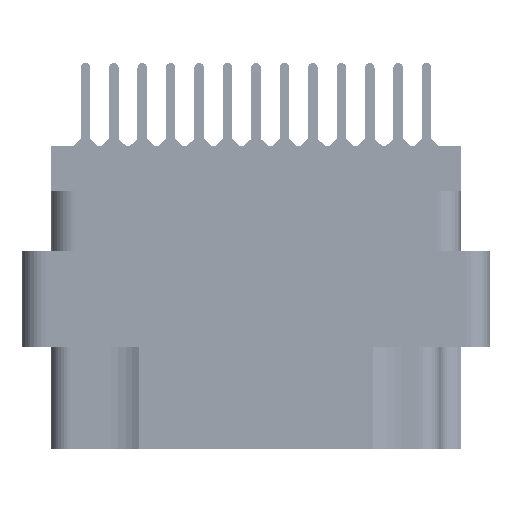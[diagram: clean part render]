
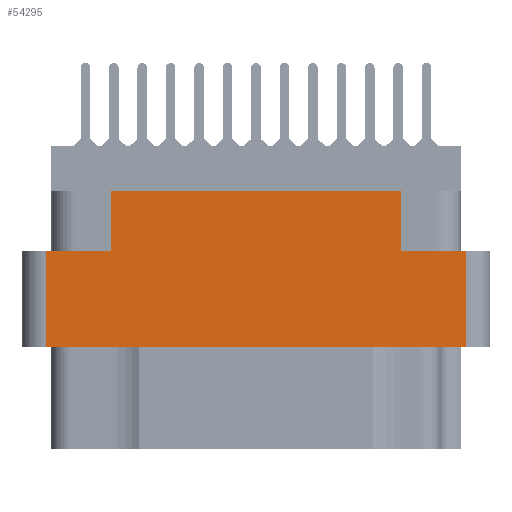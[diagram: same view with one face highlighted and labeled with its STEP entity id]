
A CAD part, left-side view. The second image highlights one B-rep face of the part: STEP entity #54295.
In plain terms, the highlighted planar face has unit normal (-1, 0, 0).
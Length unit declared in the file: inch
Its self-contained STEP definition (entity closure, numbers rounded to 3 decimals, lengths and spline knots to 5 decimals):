
#171 = DIRECTION ( 'NONE',  ( 0., 0., 1. ) ) ;
#1696 = LINE ( 'NONE', #37848, #60438 ) ;
#2802 = CARTESIAN_POINT ( 'NONE',  ( -1.359, -0.555, -0.798 ) ) ;
#3169 = VERTEX_POINT ( 'NONE', #52863 ) ;
#4063 = CARTESIAN_POINT ( 'NONE',  ( -1.359, 0.555, -0.798 ) ) ;
#6228 = LINE ( 'NONE', #41258, #57355 ) ;
#6602 = CARTESIAN_POINT ( 'NONE',  ( -1.359, -0.3825, -0.277 ) ) ;
#6632 = ORIENTED_EDGE ( 'NONE', *, *, #34053, .F. ) ;
#7445 = CARTESIAN_POINT ( 'NONE',  ( -1.359, -0.555, -0.277 ) ) ;
#7615 = ORIENTED_EDGE ( 'NONE', *, *, #39332, .F. ) ;
#7679 = VERTEX_POINT ( 'NONE', #59091 ) ;
#8671 = CARTESIAN_POINT ( 'NONE',  ( -1.359, 0.555, -0.529 ) ) ;
#9041 = DIRECTION ( 'NONE',  ( 0., 0., 1. ) ) ;
#10512 = EDGE_CURVE ( 'NONE', #35451, #7679, #48412, .T. ) ;
#11141 = LINE ( 'NONE', #4063, #49497 ) ;
#13252 = AXIS2_PLACEMENT_3D ( 'NONE', #14838, #52762, #20114 ) ;
#13747 = EDGE_CURVE ( 'NONE', #23393, #40418, #6228, .T. ) ;
#14532 = DIRECTION ( 'NONE',  ( 0., 0., -1. ) ) ;
#14607 = PLANE ( 'NONE',  #13252 ) ;
#14838 = CARTESIAN_POINT ( 'NONE',  ( -1.359, -0.617, -0.798 ) ) ;
#17220 = VERTEX_POINT ( 'NONE', #7445 ) ;
#19084 = LINE ( 'NONE', #23285, #31061 ) ;
#20112 = EDGE_CURVE ( 'NONE', #23393, #17220, #23311, .T. ) ;
#20114 = DIRECTION ( 'NONE',  ( 0., 0., 1. ) ) ;
#20311 = EDGE_CURVE ( 'NONE', #35451, #17220, #59917, .T. ) ;
#23285 = CARTESIAN_POINT ( 'NONE',  ( -1.359, 0., -0.277 ) ) ;
#23311 = LINE ( 'NONE', #2802, #70153 ) ;
#23393 = VERTEX_POINT ( 'NONE', #26243 ) ;
#26243 = CARTESIAN_POINT ( 'NONE',  ( -1.359, -0.555, -0.529 ) ) ;
#28966 = ORIENTED_EDGE ( 'NONE', *, *, #10512, .T. ) ;
#29539 = EDGE_LOOP ( 'NONE', ( #6632, #41146, #60265, #61091, #62860, #28966, #7615, #56392 ) ) ;
#30198 = VERTEX_POINT ( 'NONE', #33476 ) ;
#31061 = VECTOR ( 'NONE', #45719, 39.37008 ) ;
#33433 = VERTEX_POINT ( 'NONE', #57654 ) ;
#33476 = CARTESIAN_POINT ( 'NONE',  ( -1.359, 0.555, -0.277 ) ) ;
#34053 = EDGE_CURVE ( 'NONE', #30198, #33433, #19084, .T. ) ;
#35451 = VERTEX_POINT ( 'NONE', #6602 ) ;
#37834 = CARTESIAN_POINT ( 'NONE',  ( -1.359, 0., -0.277 ) ) ;
#37848 = CARTESIAN_POINT ( 'NONE',  ( -1.359, 0.617, -0.117 ) ) ;
#38007 = EDGE_CURVE ( 'NONE', #33433, #3169, #68318, .T. ) ;
#39332 = EDGE_CURVE ( 'NONE', #3169, #7679, #1696, .T. ) ;
#40418 = VERTEX_POINT ( 'NONE', #8671 ) ;
#41146 = ORIENTED_EDGE ( 'NONE', *, *, #47521, .T. ) ;
#41258 = CARTESIAN_POINT ( 'NONE',  ( -1.359, 0., -0.529 ) ) ;
#43101 = DIRECTION ( 'NONE',  ( 0., -1., 0. ) ) ;
#44653 = VECTOR ( 'NONE', #70182, 39.37008 ) ;
#45719 = DIRECTION ( 'NONE',  ( 0., -1., 0. ) ) ;
#46242 = VECTOR ( 'NONE', #171, 39.37008 ) ;
#47521 = EDGE_CURVE ( 'NONE', #30198, #40418, #11141, .T. ) ;
#48412 = LINE ( 'NONE', #62634, #67168 ) ;
#49497 = VECTOR ( 'NONE', #14532, 39.37008 ) ;
#51963 = DIRECTION ( 'NONE',  ( 0., 0., 1. ) ) ;
#52504 = FACE_OUTER_BOUND ( 'NONE', #29539, .T. ) ;
#52762 = DIRECTION ( 'NONE',  ( -1., 0., 0. ) ) ;
#52863 = CARTESIAN_POINT ( 'NONE',  ( -1.359, 0.3825, -0.117 ) ) ;
#54021 = CARTESIAN_POINT ( 'NONE',  ( -1.359, 0.3825, -0.277 ) ) ;
#54295 = ADVANCED_FACE ( 'NONE', ( #52504 ), #14607, .T. ) ;
#56392 = ORIENTED_EDGE ( 'NONE', *, *, #38007, .F. ) ;
#56946 = DIRECTION ( 'NONE',  ( 0., 1., 0. ) ) ;
#57355 = VECTOR ( 'NONE', #56946, 39.37008 ) ;
#57654 = CARTESIAN_POINT ( 'NONE',  ( -1.359, 0.3825, -0.277 ) ) ;
#59091 = CARTESIAN_POINT ( 'NONE',  ( -1.359, -0.3825, -0.117 ) ) ;
#59917 = LINE ( 'NONE', #37834, #44653 ) ;
#60265 = ORIENTED_EDGE ( 'NONE', *, *, #13747, .F. ) ;
#60438 = VECTOR ( 'NONE', #43101, 39.37008 ) ;
#61091 = ORIENTED_EDGE ( 'NONE', *, *, #20112, .T. ) ;
#62634 = CARTESIAN_POINT ( 'NONE',  ( -1.359, -0.3825, -0.277 ) ) ;
#62860 = ORIENTED_EDGE ( 'NONE', *, *, #20311, .F. ) ;
#67168 = VECTOR ( 'NONE', #51963, 39.37008 ) ;
#68318 = LINE ( 'NONE', #54021, #46242 ) ;
#70153 = VECTOR ( 'NONE', #9041, 39.37008 ) ;
#70182 = DIRECTION ( 'NONE',  ( 0., -1., 0. ) ) ;
